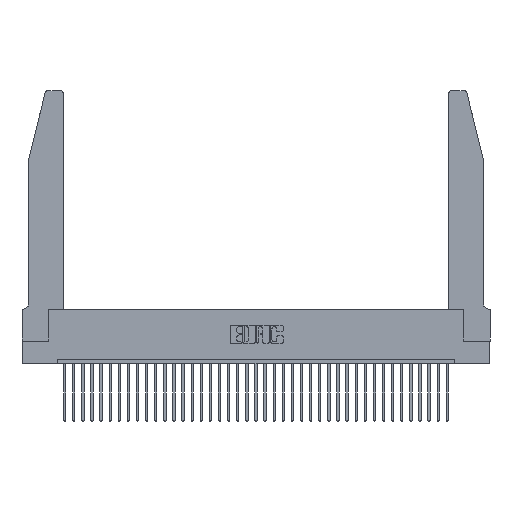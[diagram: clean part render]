
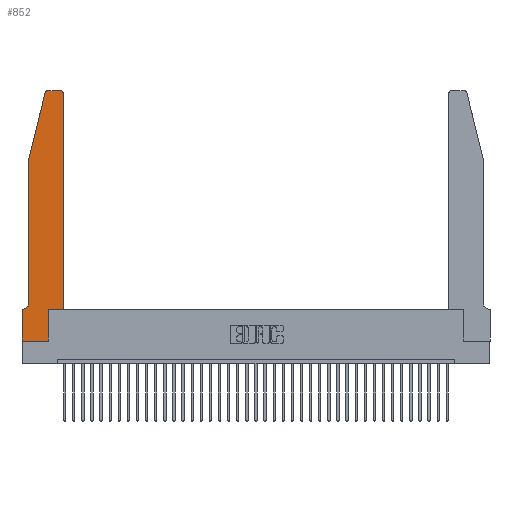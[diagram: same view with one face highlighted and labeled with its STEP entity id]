
A CAD part, top view. The second image highlights one B-rep face of the part: STEP entity #852.
In plain terms, the highlighted planar face has unit normal (0, 0, 1).
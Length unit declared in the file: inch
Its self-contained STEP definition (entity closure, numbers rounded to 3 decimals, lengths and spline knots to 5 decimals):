
#852 = ADVANCED_FACE ( 'NONE', ( #27145 ), #5231, .T. ) ;
#898 = CARTESIAN_POINT ( 'NONE',  ( 0.2865, 0.35, 0.37 ) ) ;
#1014 = DIRECTION ( 'NONE',  ( 0., 0., 1. ) ) ;
#1150 = DIRECTION ( 'NONE',  ( 1., 0., 0. ) ) ;
#1281 = VERTEX_POINT ( 'NONE', #10363 ) ;
#1920 = DIRECTION ( 'NONE',  ( 0., 0., -1. ) ) ;
#2062 = CARTESIAN_POINT ( 'NONE',  ( 0., 0., 0.37 ) ) ;
#2315 = CARTESIAN_POINT ( 'NONE',  ( 0., 0., 0.37 ) ) ;
#2458 = VECTOR ( 'NONE', #29086, 39.37008 ) ;
#2534 = LINE ( 'NONE', #2062, #4320 ) ;
#3509 = CARTESIAN_POINT ( 'NONE',  ( 0.284, 2.72, 0.37 ) ) ;
#4171 = VERTEX_POINT ( 'NONE', #33783 ) ;
#4320 = VECTOR ( 'NONE', #7507, 39.37008 ) ;
#4336 = EDGE_CURVE ( 'NONE', #26714, #10122, #20631, .T. ) ;
#4869 = VERTEX_POINT ( 'NONE', #2315 ) ;
#5095 = ORIENTED_EDGE ( 'NONE', *, *, #26297, .T. ) ;
#5231 = PLANE ( 'NONE',  #21599 ) ;
#5302 = CARTESIAN_POINT ( 'NONE',  ( 0.4505, 0.35, 0.37 ) ) ;
#5422 = ORIENTED_EDGE ( 'NONE', *, *, #18014, .T. ) ;
#5573 = EDGE_CURVE ( 'NONE', #1281, #26714, #20511, .T. ) ;
#6131 = EDGE_CURVE ( 'NONE', #26201, #13048, #24793, .T. ) ;
#6182 = DIRECTION ( 'NONE',  ( 1., 0., 0. ) ) ;
#6403 = LINE ( 'NONE', #34387, #2458 ) ;
#6815 = DIRECTION ( 'NONE',  ( 0., -1., 0. ) ) ;
#7507 = DIRECTION ( 'NONE',  ( 1., 0., 0. ) ) ;
#7984 = VERTEX_POINT ( 'NONE', #24254 ) ;
#8417 = CARTESIAN_POINT ( 'NONE',  ( 0., 0., 0.37 ) ) ;
#9177 = EDGE_CURVE ( 'NONE', #24266, #1281, #28363, .T. ) ;
#9770 = DIRECTION ( 'NONE',  ( 1., 0., 0. ) ) ;
#10090 = VECTOR ( 'NONE', #12992, 39.37008 ) ;
#10122 = VERTEX_POINT ( 'NONE', #13396 ) ;
#10363 = CARTESIAN_POINT ( 'NONE',  ( 0.4505, 2.72, 0.37 ) ) ;
#10570 = VECTOR ( 'NONE', #13668, 39.37008 ) ;
#10643 = VECTOR ( 'NONE', #12436, 39.37008 ) ;
#11372 = CARTESIAN_POINT ( 'NONE',  ( 0.4505, 0.35, 0.37 ) ) ;
#11786 = LINE ( 'NONE', #8417, #25198 ) ;
#11796 = VERTEX_POINT ( 'NONE', #18099 ) ;
#12128 = CIRCLE ( 'NONE', #14270, 0.07 ) ;
#12436 = DIRECTION ( 'NONE',  ( -1., 0., 0. ) ) ;
#12992 = DIRECTION ( 'NONE',  ( -0.239, -0.971, 0. ) ) ;
#13048 = VERTEX_POINT ( 'NONE', #34108 ) ;
#13396 = CARTESIAN_POINT ( 'NONE',  ( 0.284, 2.75, 0.37 ) ) ;
#13453 = DIRECTION ( 'NONE',  ( -1., 0., 0. ) ) ;
#13668 = DIRECTION ( 'NONE',  ( 0., 1., 0. ) ) ;
#14057 = DIRECTION ( 'NONE',  ( 0., 0., 1. ) ) ;
#14122 = CARTESIAN_POINT ( 'NONE',  ( 0.4205, 2.75, 0.37 ) ) ;
#14159 = CARTESIAN_POINT ( 'NONE',  ( 0., 0.35, 0.37 ) ) ;
#14270 = AXIS2_PLACEMENT_3D ( 'NONE', #33209, #1920, #33467 ) ;
#14322 = ORIENTED_EDGE ( 'NONE', *, *, #6131, .T. ) ;
#15388 = EDGE_CURVE ( 'NONE', #11796, #7984, #12128, .T. ) ;
#15553 = CARTESIAN_POINT ( 'NONE',  ( 0.0755, 0.35, 0.37 ) ) ;
#16444 = ORIENTED_EDGE ( 'NONE', *, *, #29999, .T. ) ;
#16458 = CARTESIAN_POINT ( 'NONE',  ( 0.25487, 2.72718, 0.37 ) ) ;
#17217 = EDGE_LOOP ( 'NONE', ( #17384, #29355, #14322, #34266, #19498, #24959, #5095, #5422, #16444, #27523, #34405, #21029 ) ) ;
#17384 = ORIENTED_EDGE ( 'NONE', *, *, #4336, .T. ) ;
#18014 = EDGE_CURVE ( 'NONE', #4869, #4171, #2534, .T. ) ;
#18049 = CARTESIAN_POINT ( 'NONE',  ( 0.0755, 2., 0.37 ) ) ;
#18099 = CARTESIAN_POINT ( 'NONE',  ( 0.0755, 0.42, 0.37 ) ) ;
#19402 = VECTOR ( 'NONE', #6815, 39.37008 ) ;
#19498 = ORIENTED_EDGE ( 'NONE', *, *, #15388, .T. ) ;
#19766 = VECTOR ( 'NONE', #13453, 39.37008 ) ;
#20511 = CIRCLE ( 'NONE', #28600, 0.03 ) ;
#20529 = CARTESIAN_POINT ( 'NONE',  ( 0.4505, 0.35, 0.37 ) ) ;
#20631 = LINE ( 'NONE', #33423, #19766 ) ;
#21029 = ORIENTED_EDGE ( 'NONE', *, *, #5573, .T. ) ;
#21599 = AXIS2_PLACEMENT_3D ( 'NONE', #31317, #14057, #22282 ) ;
#21880 = VERTEX_POINT ( 'NONE', #898 ) ;
#22282 = DIRECTION ( 'NONE',  ( 1., 0., 0. ) ) ;
#22968 = VECTOR ( 'NONE', #6182, 39.37008 ) ;
#23420 = LINE ( 'NONE', #20529, #22968 ) ;
#24254 = CARTESIAN_POINT ( 'NONE',  ( 0.0055, 0.35, 0.37 ) ) ;
#24266 = VERTEX_POINT ( 'NONE', #11372 ) ;
#24793 = LINE ( 'NONE', #29774, #10090 ) ;
#24959 = ORIENTED_EDGE ( 'NONE', *, *, #34504, .T. ) ;
#25198 = VECTOR ( 'NONE', #25860, 39.37008 ) ;
#25362 = LINE ( 'NONE', #15553, #10643 ) ;
#25506 = AXIS2_PLACEMENT_3D ( 'NONE', #3509, #1014, #1150 ) ;
#25735 = EDGE_CURVE ( 'NONE', #21880, #24266, #23420, .T. ) ;
#25860 = DIRECTION ( 'NONE',  ( 0., -1., 0. ) ) ;
#26201 = VERTEX_POINT ( 'NONE', #16458 ) ;
#26297 = EDGE_CURVE ( 'NONE', #34852, #4869, #11786, .T. ) ;
#26714 = VERTEX_POINT ( 'NONE', #14122 ) ;
#26924 = EDGE_CURVE ( 'NONE', #10122, #26201, #30004, .T. ) ;
#27145 = FACE_OUTER_BOUND ( 'NONE', #17217, .T. ) ;
#27523 = ORIENTED_EDGE ( 'NONE', *, *, #25735, .T. ) ;
#28363 = LINE ( 'NONE', #5302, #10570 ) ;
#28600 = AXIS2_PLACEMENT_3D ( 'NONE', #28910, #32166, #9770 ) ;
#28910 = CARTESIAN_POINT ( 'NONE',  ( 0.4205, 2.72, 0.37 ) ) ;
#29086 = DIRECTION ( 'NONE',  ( 0., 1., 0. ) ) ;
#29355 = ORIENTED_EDGE ( 'NONE', *, *, #26924, .T. ) ;
#29774 = CARTESIAN_POINT ( 'NONE',  ( 0.0755, 2., 0.37 ) ) ;
#29999 = EDGE_CURVE ( 'NONE', #4171, #21880, #6403, .T. ) ;
#30004 = CIRCLE ( 'NONE', #25506, 0.03 ) ;
#30166 = EDGE_CURVE ( 'NONE', #13048, #11796, #34533, .T. ) ;
#31317 = CARTESIAN_POINT ( 'NONE',  ( 0., 0.35, 0.37 ) ) ;
#32166 = DIRECTION ( 'NONE',  ( 0., 0., 1. ) ) ;
#33209 = CARTESIAN_POINT ( 'NONE',  ( 0.0055, 0.42, 0.37 ) ) ;
#33423 = CARTESIAN_POINT ( 'NONE',  ( 0.2605, 2.75, 0.37 ) ) ;
#33467 = DIRECTION ( 'NONE',  ( -1., 0., 0. ) ) ;
#33783 = CARTESIAN_POINT ( 'NONE',  ( 0.2865, 0., 0.37 ) ) ;
#34108 = CARTESIAN_POINT ( 'NONE',  ( 0.0755, 2., 0.37 ) ) ;
#34266 = ORIENTED_EDGE ( 'NONE', *, *, #30166, .T. ) ;
#34387 = CARTESIAN_POINT ( 'NONE',  ( 0.2865, 0.35, 0.37 ) ) ;
#34405 = ORIENTED_EDGE ( 'NONE', *, *, #9177, .T. ) ;
#34504 = EDGE_CURVE ( 'NONE', #7984, #34852, #25362, .T. ) ;
#34533 = LINE ( 'NONE', #18049, #19402 ) ;
#34852 = VERTEX_POINT ( 'NONE', #14159 ) ;
